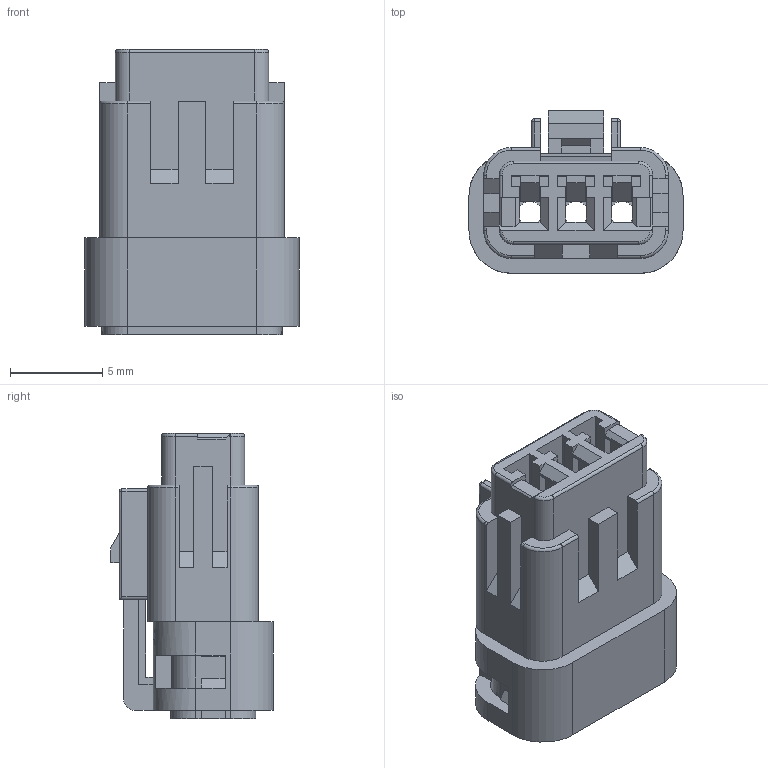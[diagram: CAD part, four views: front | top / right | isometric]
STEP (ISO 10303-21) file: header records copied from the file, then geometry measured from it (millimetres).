
FILE_DESCRIPTION (( 'STEP AP214' ), '1' );
FILE_NAME ('565-003-000-411.STEP', '2020-07-27T15:36:43', ( '' ), ( '' ), 'SwSTEP 2.0', 'SolidWorks 2020', '' );
FILE_SCHEMA (( 'AUTOMOTIVE_DESIGN' ));
Length unit declared in the file: millimetre
Products named in the file (4): 565-003-000-411; 565-003-000-411_Housing; 565-003-000-411_Rear Gasket; 565-003-000-411_Rear Insulator
Assembly tree (3 placements, depth 2):
  565-003-000-411
    565-003-000-411_Housing
    565-003-000-411_Rear Insulator
    565-003-000-411_Rear Gasket
Bounding box: 11.6 x 8.8 x 15.44 mm (x, y, z)
Volume: 659.4 mm3; surface area: 1718.3 mm2
Topology: 5 solids, 5 shells, 377 faces, 1048 edges, 685 vertices
Faces by surface type: plane 257, cylinder 86, torus 18, bspline 14, sphere 2
Entity records: 12785 total; most frequent: CARTESIAN_POINT 2872, ORIENTED_EDGE 2092, DIRECTION 1951, EDGE_CURVE 1046, LINE 779, VECTOR 779, VERTEX_POINT 685, AXIS2_PLACEMENT_3D 586
